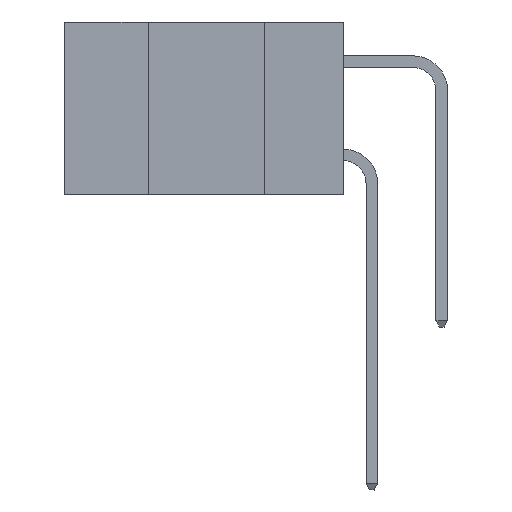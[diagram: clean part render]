
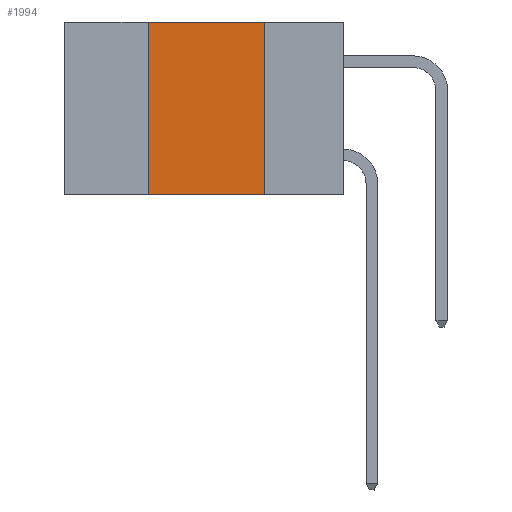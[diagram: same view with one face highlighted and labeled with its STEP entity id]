
A CAD part, left-side view. The second image highlights one B-rep face of the part: STEP entity #1994.
In plain terms, the highlighted planar face has unit normal (-1, 0, 0).
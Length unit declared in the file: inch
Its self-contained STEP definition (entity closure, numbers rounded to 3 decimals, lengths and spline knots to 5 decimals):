
#400 = VECTOR ( 'NONE', #12628, 39.37008 ) ;
#464 = VECTOR ( 'NONE', #2688, 39.37008 ) ;
#1034 = CARTESIAN_POINT ( 'NONE',  ( 0., 0.42, -0.37 ) ) ;
#1134 = DIRECTION ( 'NONE',  ( 1., 0., 0. ) ) ;
#1686 = CARTESIAN_POINT ( 'NONE',  ( 0., 0.17, -0.37 ) ) ;
#1883 = ORIENTED_EDGE ( 'NONE', *, *, #2226, .T. ) ;
#1913 = DIRECTION ( 'NONE',  ( 0., -1., 0. ) ) ;
#1994 = ADVANCED_FACE ( 'NONE', ( #9769 ), #10884, .F. ) ;
#2226 = EDGE_CURVE ( 'NONE', #14816, #7872, #12767, .T. ) ;
#2373 = CARTESIAN_POINT ( 'NONE',  ( 0., 0.17, -0.37 ) ) ;
#2474 = DIRECTION ( 'NONE',  ( 0., -1., 0. ) ) ;
#2688 = DIRECTION ( 'NONE',  ( 0., 0., 1. ) ) ;
#2884 = CARTESIAN_POINT ( 'NONE',  ( 0., 0.17, 0. ) ) ;
#4040 = LINE ( 'NONE', #10044, #464 ) ;
#6228 = VERTEX_POINT ( 'NONE', #11311 ) ;
#6260 = LINE ( 'NONE', #1686, #400 ) ;
#7451 = AXIS2_PLACEMENT_3D ( 'NONE', #10727, #1134, #14600 ) ;
#7872 = VERTEX_POINT ( 'NONE', #2373 ) ;
#8213 = ORIENTED_EDGE ( 'NONE', *, *, #13053, .F. ) ;
#8414 = EDGE_CURVE ( 'NONE', #10981, #7872, #6260, .T. ) ;
#8623 = LINE ( 'NONE', #13392, #13881 ) ;
#9381 = EDGE_CURVE ( 'NONE', #6228, #10981, #8623, .T. ) ;
#9769 = FACE_OUTER_BOUND ( 'NONE', #14966, .T. ) ;
#9869 = VECTOR ( 'NONE', #1913, 39.37008 ) ;
#10044 = CARTESIAN_POINT ( 'NONE',  ( 0., 0.42, -0.37 ) ) ;
#10309 = CARTESIAN_POINT ( 'NONE',  ( 0., 0.6, -0.37 ) ) ;
#10727 = CARTESIAN_POINT ( 'NONE',  ( 0., 0.6, 0. ) ) ;
#10733 = ORIENTED_EDGE ( 'NONE', *, *, #8414, .F. ) ;
#10884 = PLANE ( 'NONE',  #7451 ) ;
#10981 = VERTEX_POINT ( 'NONE', #2884 ) ;
#11311 = CARTESIAN_POINT ( 'NONE',  ( 0., 0.42, 0. ) ) ;
#12628 = DIRECTION ( 'NONE',  ( 0., 0., -1. ) ) ;
#12767 = LINE ( 'NONE', #10309, #9869 ) ;
#13053 = EDGE_CURVE ( 'NONE', #14816, #6228, #4040, .T. ) ;
#13392 = CARTESIAN_POINT ( 'NONE',  ( 0., 0.6, 0. ) ) ;
#13881 = VECTOR ( 'NONE', #2474, 39.37008 ) ;
#14382 = ORIENTED_EDGE ( 'NONE', *, *, #9381, .F. ) ;
#14600 = DIRECTION ( 'NONE',  ( 0., 0., -1. ) ) ;
#14816 = VERTEX_POINT ( 'NONE', #1034 ) ;
#14966 = EDGE_LOOP ( 'NONE', ( #10733, #14382, #8213, #1883 ) ) ;
